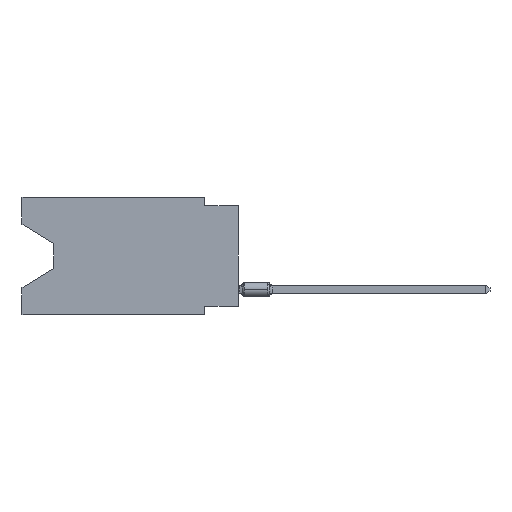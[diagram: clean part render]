
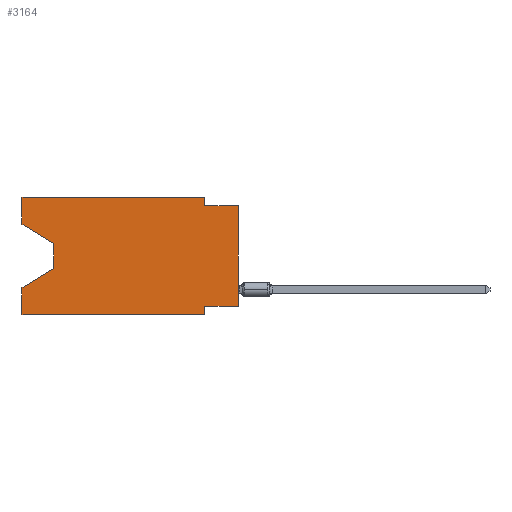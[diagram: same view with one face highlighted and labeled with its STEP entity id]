
A CAD part, left-side view. The second image highlights one B-rep face of the part: STEP entity #3164.
In plain terms, the highlighted planar face has unit normal (-1, 0, 0).
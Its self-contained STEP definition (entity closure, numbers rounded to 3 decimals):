
#1540 = VERTEX_POINT ( 'NONE', #1953 ) ;
#1577 = VERTEX_POINT ( 'NONE', #18228 ) ;
#1893 = EDGE_LOOP ( 'NONE', ( #16964, #8333, #18994, #19936, #3960, #15337, #6760, #26476, #20402, #30105, #22747, #26430 ) ) ;
#1922 = VERTEX_POINT ( 'NONE', #9964 ) ;
#1953 = CARTESIAN_POINT ( 'NONE',  ( 0., 13.97, -5.385 ) ) ;
#2303 = VECTOR ( 'NONE', #20680, 1000. ) ;
#2832 = DIRECTION ( 'NONE',  ( 0., -1., 0. ) ) ;
#2997 = EDGE_CURVE ( 'NONE', #21219, #18885, #15815, .T. ) ;
#3051 = EDGE_CURVE ( 'NONE', #21764, #1577, #33970, .T. ) ;
#3130 = DIRECTION ( 'NONE',  ( 0., -0.855, -0.519 ) ) ;
#3164 = ADVANCED_FACE ( 'NONE', ( #16502 ), #24000, .F. ) ;
#3183 = DIRECTION ( 'NONE',  ( 1., 0., 0. ) ) ;
#3325 = DIRECTION ( 'NONE',  ( 0., 0., -1. ) ) ;
#3752 = CARTESIAN_POINT ( 'NONE',  ( 0., 16.383, -8.89 ) ) ;
#3960 = ORIENTED_EDGE ( 'NONE', *, *, #3051, .T. ) ;
#4430 = VECTOR ( 'NONE', #4607, 1000. ) ;
#4472 = LINE ( 'NONE', #23012, #20797 ) ;
#4559 = DIRECTION ( 'NONE',  ( 0., 0.855, -0.519 ) ) ;
#4607 = DIRECTION ( 'NONE',  ( 0., -1., 0. ) ) ;
#5127 = DIRECTION ( 'NONE',  ( 0., 0., -1. ) ) ;
#6122 = CARTESIAN_POINT ( 'NONE',  ( 0., 2.54, -8.89 ) ) ;
#6760 = ORIENTED_EDGE ( 'NONE', *, *, #9836, .F. ) ;
#6966 = LINE ( 'NONE', #17655, #7733 ) ;
#7227 = CARTESIAN_POINT ( 'NONE',  ( 0., 2.54, 0. ) ) ;
#7733 = VECTOR ( 'NONE', #33184, 1000. ) ;
#7845 = VECTOR ( 'NONE', #3325, 1000. ) ;
#8333 = ORIENTED_EDGE ( 'NONE', *, *, #15593, .T. ) ;
#9149 = CARTESIAN_POINT ( 'NONE',  ( 0., 0., -8.255 ) ) ;
#9649 = LINE ( 'NONE', #30780, #2303 ) ;
#9836 = EDGE_CURVE ( 'NONE', #10052, #1922, #16009, .T. ) ;
#9964 = CARTESIAN_POINT ( 'NONE',  ( 0., 2.54, -8.255 ) ) ;
#10052 = VERTEX_POINT ( 'NONE', #9149 ) ;
#10401 = VECTOR ( 'NONE', #3130, 1000. ) ;
#11177 = VECTOR ( 'NONE', #5127, 1000. ) ;
#11326 = CARTESIAN_POINT ( 'NONE',  ( 0., 0., -0.635 ) ) ;
#11764 = EDGE_CURVE ( 'NONE', #12643, #12511, #4472, .T. ) ;
#11839 = CARTESIAN_POINT ( 'NONE',  ( 0., 16.383, -6.852 ) ) ;
#12511 = VERTEX_POINT ( 'NONE', #26612 ) ;
#12643 = VERTEX_POINT ( 'NONE', #14725 ) ;
#13377 = CARTESIAN_POINT ( 'NONE',  ( 0., 2.54, 0. ) ) ;
#13874 = DIRECTION ( 'NONE',  ( 0., 0., -1. ) ) ;
#14339 = CARTESIAN_POINT ( 'NONE',  ( 0., 16.383, -2.038 ) ) ;
#14573 = VERTEX_POINT ( 'NONE', #11839 ) ;
#14725 = CARTESIAN_POINT ( 'NONE',  ( 0., 16.383, -2.038 ) ) ;
#15071 = CARTESIAN_POINT ( 'NONE',  ( 0., 13.97, -5.385 ) ) ;
#15337 = ORIENTED_EDGE ( 'NONE', *, *, #30445, .F. ) ;
#15593 = EDGE_CURVE ( 'NONE', #33958, #1540, #25986, .T. ) ;
#15815 = LINE ( 'NONE', #7227, #11177 ) ;
#16009 = LINE ( 'NONE', #18982, #16811 ) ;
#16502 = FACE_OUTER_BOUND ( 'NONE', #1893, .T. ) ;
#16811 = VECTOR ( 'NONE', #21421, 1000. ) ;
#16964 = ORIENTED_EDGE ( 'NONE', *, *, #26643, .T. ) ;
#17655 = CARTESIAN_POINT ( 'NONE',  ( 0., 0., -0.635 ) ) ;
#18228 = CARTESIAN_POINT ( 'NONE',  ( 0., 2.54, -8.89 ) ) ;
#18438 = VECTOR ( 'NONE', #2832, 1000. ) ;
#18439 = VERTEX_POINT ( 'NONE', #11326 ) ;
#18505 = LINE ( 'NONE', #29131, #28786 ) ;
#18777 = CARTESIAN_POINT ( 'NONE',  ( 0., 16.383, 0. ) ) ;
#18885 = VERTEX_POINT ( 'NONE', #24708 ) ;
#18982 = CARTESIAN_POINT ( 'NONE',  ( 0., 0., -8.255 ) ) ;
#18994 = ORIENTED_EDGE ( 'NONE', *, *, #24024, .T. ) ;
#19189 = VECTOR ( 'NONE', #20264, 1000. ) ;
#19936 = ORIENTED_EDGE ( 'NONE', *, *, #28966, .F. ) ;
#20264 = DIRECTION ( 'NONE',  ( 0., 0., -1. ) ) ;
#20402 = ORIENTED_EDGE ( 'NONE', *, *, #25646, .F. ) ;
#20672 = EDGE_CURVE ( 'NONE', #10052, #18439, #18505, .T. ) ;
#20680 = DIRECTION ( 'NONE',  ( 0., 0., 1. ) ) ;
#20797 = VECTOR ( 'NONE', #24801, 1000. ) ;
#21219 = VERTEX_POINT ( 'NONE', #13377 ) ;
#21394 = LINE ( 'NONE', #18777, #18438 ) ;
#21421 = DIRECTION ( 'NONE',  ( 0., 1., 0. ) ) ;
#21764 = VERTEX_POINT ( 'NONE', #3752 ) ;
#22747 = ORIENTED_EDGE ( 'NONE', *, *, #27499, .F. ) ;
#23012 = CARTESIAN_POINT ( 'NONE',  ( 0., 16.383, 0. ) ) ;
#23499 = CARTESIAN_POINT ( 'NONE',  ( 0., 16.383, -8.89 ) ) ;
#24000 = PLANE ( 'NONE',  #33816 ) ;
#24024 = EDGE_CURVE ( 'NONE', #1540, #14573, #25702, .T. ) ;
#24708 = CARTESIAN_POINT ( 'NONE',  ( 0., 2.54, -0.635 ) ) ;
#24801 = DIRECTION ( 'NONE',  ( 0., 0., 1. ) ) ;
#25646 = EDGE_CURVE ( 'NONE', #18885, #18439, #6966, .T. ) ;
#25702 = LINE ( 'NONE', #15071, #28365 ) ;
#25986 = LINE ( 'NONE', #33323, #19189 ) ;
#26430 = ORIENTED_EDGE ( 'NONE', *, *, #11764, .F. ) ;
#26476 = ORIENTED_EDGE ( 'NONE', *, *, #20672, .T. ) ;
#26612 = CARTESIAN_POINT ( 'NONE',  ( 0., 16.383, 0. ) ) ;
#26643 = EDGE_CURVE ( 'NONE', #12643, #33958, #27245, .T. ) ;
#27124 = CARTESIAN_POINT ( 'NONE',  ( 0., 16.383, 0. ) ) ;
#27245 = LINE ( 'NONE', #14339, #10401 ) ;
#27499 = EDGE_CURVE ( 'NONE', #12511, #21219, #21394, .T. ) ;
#28365 = VECTOR ( 'NONE', #4559, 1000. ) ;
#28786 = VECTOR ( 'NONE', #29811, 1000. ) ;
#28966 = EDGE_CURVE ( 'NONE', #21764, #14573, #9649, .T. ) ;
#29131 = CARTESIAN_POINT ( 'NONE',  ( 0., 0., 0. ) ) ;
#29811 = DIRECTION ( 'NONE',  ( 0., 0., 1. ) ) ;
#30105 = ORIENTED_EDGE ( 'NONE', *, *, #2997, .F. ) ;
#30445 = EDGE_CURVE ( 'NONE', #1922, #1577, #33034, .T. ) ;
#30780 = CARTESIAN_POINT ( 'NONE',  ( 0., 16.383, 0. ) ) ;
#31491 = CARTESIAN_POINT ( 'NONE',  ( 0., 13.97, -3.505 ) ) ;
#33034 = LINE ( 'NONE', #6122, #7845 ) ;
#33184 = DIRECTION ( 'NONE',  ( 0., -1., 0. ) ) ;
#33323 = CARTESIAN_POINT ( 'NONE',  ( 0., 13.97, -3.505 ) ) ;
#33816 = AXIS2_PLACEMENT_3D ( 'NONE', #27124, #3183, #13874 ) ;
#33958 = VERTEX_POINT ( 'NONE', #31491 ) ;
#33970 = LINE ( 'NONE', #23499, #4430 ) ;
